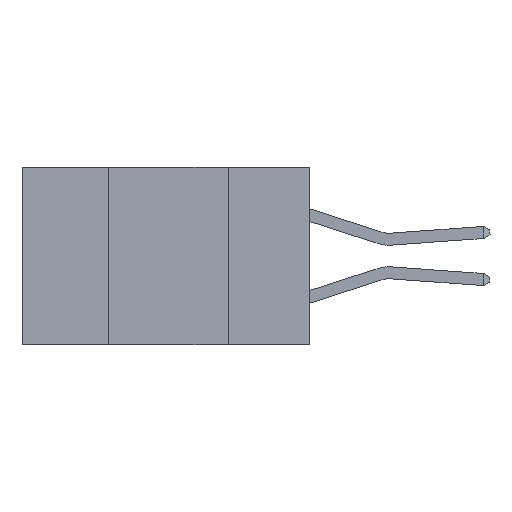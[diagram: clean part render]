
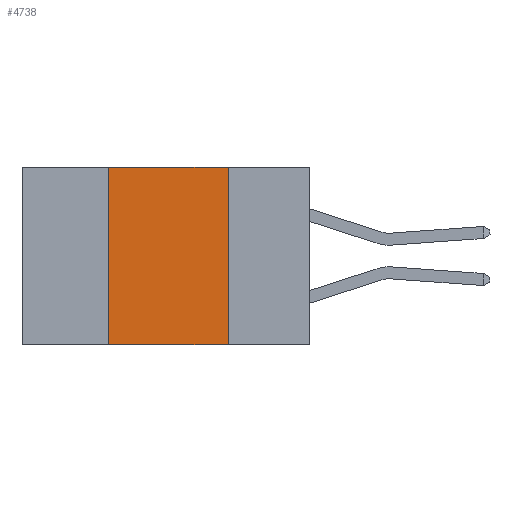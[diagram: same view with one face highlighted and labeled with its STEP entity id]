
A CAD part, left-side view. The second image highlights one B-rep face of the part: STEP entity #4738.
In plain terms, the highlighted planar face has unit normal (-1, 0, 0).
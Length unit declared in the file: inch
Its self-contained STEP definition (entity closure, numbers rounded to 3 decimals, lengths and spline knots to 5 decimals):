
#472 = CARTESIAN_POINT ( 'NONE',  ( 0., 0.42, -0.37 ) ) ;
#751 = VECTOR ( 'NONE', #12363, 39.37008 ) ;
#811 = LINE ( 'NONE', #14598, #9199 ) ;
#2280 = DIRECTION ( 'NONE',  ( 0., -1., 0. ) ) ;
#2509 = CARTESIAN_POINT ( 'NONE',  ( 0., 0.6, 0. ) ) ;
#3081 = VECTOR ( 'NONE', #16520, 39.37008 ) ;
#3391 = ORIENTED_EDGE ( 'NONE', *, *, #8592, .F. ) ;
#3975 = VERTEX_POINT ( 'NONE', #18813 ) ;
#4696 = ORIENTED_EDGE ( 'NONE', *, *, #20385, .T. ) ;
#4738 = ADVANCED_FACE ( 'NONE', ( #12302 ), #15023, .F. ) ;
#5450 = CARTESIAN_POINT ( 'NONE',  ( 0., 0.17, 0. ) ) ;
#5480 = LINE ( 'NONE', #5450, #751 ) ;
#5550 = EDGE_CURVE ( 'NONE', #16868, #3975, #18423, .T. ) ;
#6749 = EDGE_CURVE ( 'NONE', #14480, #16868, #11955, .T. ) ;
#7582 = ORIENTED_EDGE ( 'NONE', *, *, #6749, .F. ) ;
#8592 = EDGE_CURVE ( 'NONE', #3975, #12138, #5480, .T. ) ;
#9021 = CARTESIAN_POINT ( 'NONE',  ( 0., 0.42, 0. ) ) ;
#9199 = VECTOR ( 'NONE', #2280, 39.37008 ) ;
#9318 = ORIENTED_EDGE ( 'NONE', *, *, #5550, .F. ) ;
#10824 = AXIS2_PLACEMENT_3D ( 'NONE', #11755, #12535, #12505 ) ;
#11755 = CARTESIAN_POINT ( 'NONE',  ( 0., 0.6, 0. ) ) ;
#11955 = LINE ( 'NONE', #16867, #3081 ) ;
#12138 = VERTEX_POINT ( 'NONE', #17108 ) ;
#12302 = FACE_OUTER_BOUND ( 'NONE', #21390, .T. ) ;
#12363 = DIRECTION ( 'NONE',  ( 0., 0., -1. ) ) ;
#12505 = DIRECTION ( 'NONE',  ( 0., 0., -1. ) ) ;
#12535 = DIRECTION ( 'NONE',  ( 1., 0., 0. ) ) ;
#14480 = VERTEX_POINT ( 'NONE', #472 ) ;
#14598 = CARTESIAN_POINT ( 'NONE',  ( 0., 0.6, -0.37 ) ) ;
#15023 = PLANE ( 'NONE',  #10824 ) ;
#16520 = DIRECTION ( 'NONE',  ( 0., 0., 1. ) ) ;
#16867 = CARTESIAN_POINT ( 'NONE',  ( 0., 0.42, 0. ) ) ;
#16868 = VERTEX_POINT ( 'NONE', #9021 ) ;
#17108 = CARTESIAN_POINT ( 'NONE',  ( 0., 0.17, -0.37 ) ) ;
#17337 = VECTOR ( 'NONE', #19921, 39.37008 ) ;
#18423 = LINE ( 'NONE', #2509, #17337 ) ;
#18813 = CARTESIAN_POINT ( 'NONE',  ( 0., 0.17, 0. ) ) ;
#19921 = DIRECTION ( 'NONE',  ( 0., -1., 0. ) ) ;
#20385 = EDGE_CURVE ( 'NONE', #14480, #12138, #811, .T. ) ;
#21390 = EDGE_LOOP ( 'NONE', ( #3391, #9318, #7582, #4696 ) ) ;
